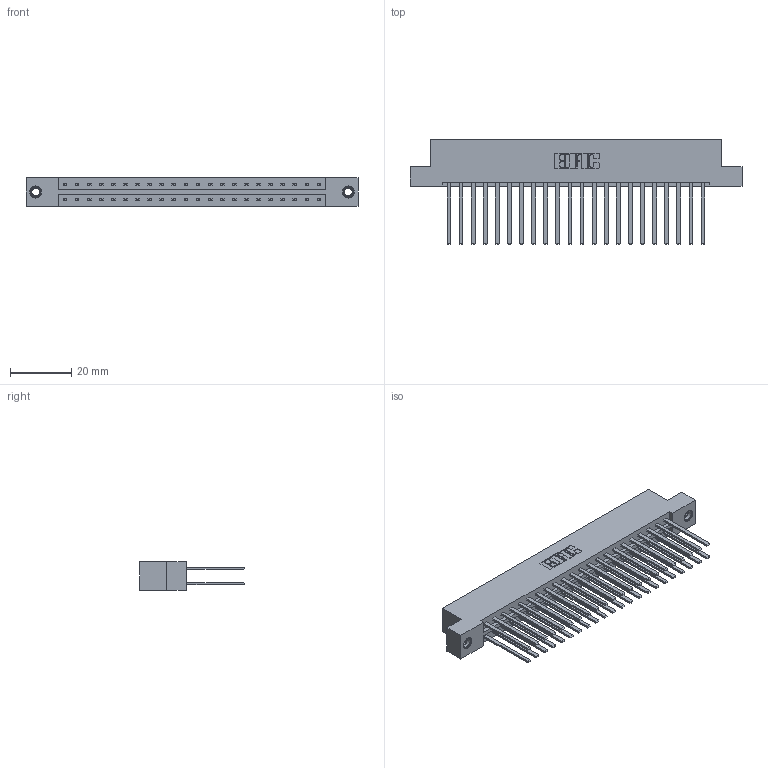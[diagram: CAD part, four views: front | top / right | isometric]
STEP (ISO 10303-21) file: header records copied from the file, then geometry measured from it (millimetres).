
FILE_DESCRIPTION (( 'STEP AP203' ), '1' );
FILE_NAME ('833-044-544-207.STEP', '2020-06-04T01:37:21', ( '' ), ( '' ), 'SwSTEP 2.0', 'SolidWorks 2020', '' );
FILE_SCHEMA (( 'CONFIG_CONTROL_DESIGN' ));
Length unit declared in the file: inch
Products named in the file (4): 833 Part_Flush - .156 Dia - TI; 833-044-544-207; 345-250-001_345-250-005-103; 345-292-001_345-293-144
Assembly tree (47 placements, depth 2):
  833-044-544-207
    833 Part_Flush - .156 Dia - TI
    345-292-001_345-293-144  x44
    345-250-001_345-250-005-103  x2
Bounding box: 108.71 x 34.3 x 9.4 mm (x, y, z)
Volume: 11515.1 mm3; surface area: 15418.9 mm2
Topology: 47 solids, 47 shells, 2198 faces, 6475 edges, 4250 vertices
Faces by surface type: plane 1510, cylinder 672, cone 12, torus 4
Entity records: 17742 total; most frequent: CARTESIAN_POINT 2945, ORIENTED_EDGE 2874, DIRECTION 2579, EDGE_CURVE 1437, LINE 1293, VECTOR 1293, VERTEX_POINT 952, AXIS2_PLACEMENT_3D 643
